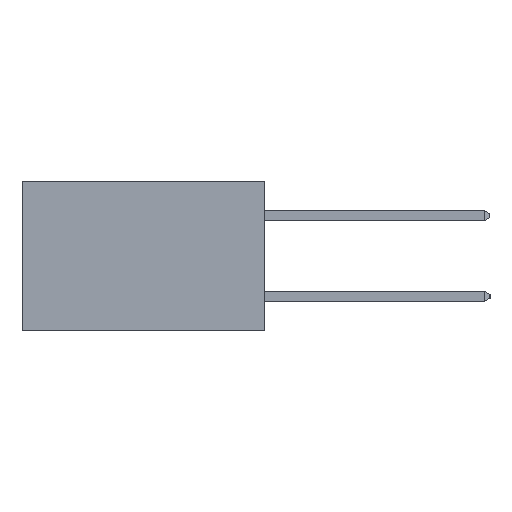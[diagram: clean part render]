
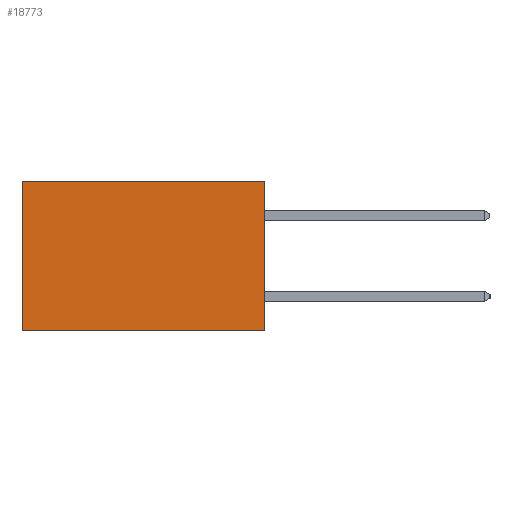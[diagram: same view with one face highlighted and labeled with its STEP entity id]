
A CAD part, left-side view. The second image highlights one B-rep face of the part: STEP entity #18773.
In plain terms, the highlighted planar face has unit normal (-1, 0, 0).
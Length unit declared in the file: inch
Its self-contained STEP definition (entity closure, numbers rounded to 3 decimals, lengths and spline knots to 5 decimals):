
#190 = CARTESIAN_POINT ( 'NONE',  ( 0.2615, 0., 0. ) ) ;
#984 = EDGE_CURVE ( 'NONE', #1816, #1039, #11852, .T. ) ;
#1039 = VERTEX_POINT ( 'NONE', #15302 ) ;
#1072 = VERTEX_POINT ( 'NONE', #4994 ) ;
#1086 = CARTESIAN_POINT ( 'NONE',  ( 0.2615, 0., 0. ) ) ;
#1816 = VERTEX_POINT ( 'NONE', #6348 ) ;
#1819 = VECTOR ( 'NONE', #10959, 39.37008 ) ;
#1862 = CARTESIAN_POINT ( 'NONE',  ( 0.2615, 0., -0.37 ) ) ;
#1972 = CARTESIAN_POINT ( 'NONE',  ( 0.2615, 0.6, -0.37 ) ) ;
#2128 = DIRECTION ( 'NONE',  ( 0., 0., -1. ) ) ;
#2734 = VERTEX_POINT ( 'NONE', #190 ) ;
#3060 = EDGE_CURVE ( 'NONE', #1072, #1039, #7446, .T. ) ;
#3434 = FACE_OUTER_BOUND ( 'NONE', #13127, .T. ) ;
#4144 = VECTOR ( 'NONE', #2128, 39.37008 ) ;
#4181 = VECTOR ( 'NONE', #15762, 39.37008 ) ;
#4994 = CARTESIAN_POINT ( 'NONE',  ( 0.2615, 0., -0.37 ) ) ;
#6348 = CARTESIAN_POINT ( 'NONE',  ( 0.2615, 0.6, 0. ) ) ;
#7446 = LINE ( 'NONE', #20607, #15605 ) ;
#7553 = CARTESIAN_POINT ( 'NONE',  ( 0.2615, 0., -0.37 ) ) ;
#8672 = ORIENTED_EDGE ( 'NONE', *, *, #984, .T. ) ;
#10169 = DIRECTION ( 'NONE',  ( 0., 0., -1. ) ) ;
#10888 = AXIS2_PLACEMENT_3D ( 'NONE', #1862, #19807, #10169 ) ;
#10959 = DIRECTION ( 'NONE',  ( 0., 1., 0. ) ) ;
#11852 = LINE ( 'NONE', #1972, #4144 ) ;
#13127 = EDGE_LOOP ( 'NONE', ( #8672, #19266, #20649, #20624 ) ) ;
#13270 = EDGE_CURVE ( 'NONE', #2734, #1816, #14926, .T. ) ;
#14926 = LINE ( 'NONE', #1086, #1819 ) ;
#15302 = CARTESIAN_POINT ( 'NONE',  ( 0.2615, 0.6, -0.37 ) ) ;
#15605 = VECTOR ( 'NONE', #20268, 39.37008 ) ;
#15762 = DIRECTION ( 'NONE',  ( 0., 0., -1. ) ) ;
#16575 = PLANE ( 'NONE',  #10888 ) ;
#17696 = LINE ( 'NONE', #7553, #4181 ) ;
#18773 = ADVANCED_FACE ( 'NONE', ( #3434 ), #16575, .F. ) ;
#19266 = ORIENTED_EDGE ( 'NONE', *, *, #3060, .F. ) ;
#19440 = EDGE_CURVE ( 'NONE', #2734, #1072, #17696, .T. ) ;
#19807 = DIRECTION ( 'NONE',  ( 1., 0., 0. ) ) ;
#20268 = DIRECTION ( 'NONE',  ( 0., 1., 0. ) ) ;
#20607 = CARTESIAN_POINT ( 'NONE',  ( 0.2615, 0., -0.37 ) ) ;
#20624 = ORIENTED_EDGE ( 'NONE', *, *, #13270, .T. ) ;
#20649 = ORIENTED_EDGE ( 'NONE', *, *, #19440, .F. ) ;
